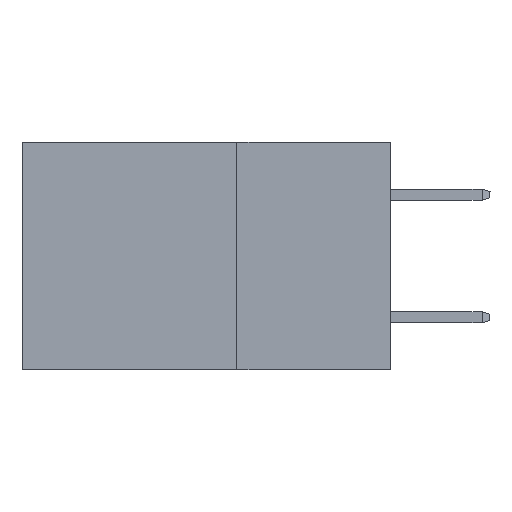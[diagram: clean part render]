
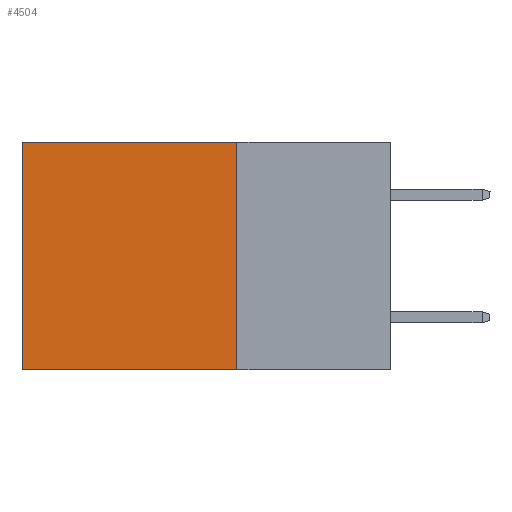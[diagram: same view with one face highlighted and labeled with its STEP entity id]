
A CAD part, left-side view. The second image highlights one B-rep face of the part: STEP entity #4504.
In plain terms, the highlighted planar face has unit normal (-1, 0, 0).
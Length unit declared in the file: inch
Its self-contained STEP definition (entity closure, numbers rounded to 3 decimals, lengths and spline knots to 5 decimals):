
#88 = VERTEX_POINT ( 'NONE', #887 ) ;
#652 = DIRECTION ( 'NONE',  ( 0., 1., 0. ) ) ;
#847 = LINE ( 'NONE', #7160, #8921 ) ;
#848 = VERTEX_POINT ( 'NONE', #3701 ) ;
#887 = CARTESIAN_POINT ( 'NONE',  ( 0.2875, 0.25, 0. ) ) ;
#898 = CARTESIAN_POINT ( 'NONE',  ( 0.2875, 0.25, -0.37 ) ) ;
#971 = ORIENTED_EDGE ( 'NONE', *, *, #4307, .T. ) ;
#2043 = EDGE_LOOP ( 'NONE', ( #971, #7208, #7688, #5482 ) ) ;
#2415 = CARTESIAN_POINT ( 'NONE',  ( 0.2875, 0.6, -0.37 ) ) ;
#2601 = LINE ( 'NONE', #8490, #6053 ) ;
#3211 = VECTOR ( 'NONE', #5764, 39.37008 ) ;
#3268 = DIRECTION ( 'NONE',  ( 0., 0., -1. ) ) ;
#3701 = CARTESIAN_POINT ( 'NONE',  ( 0.2875, 0.6, 0. ) ) ;
#4112 = VECTOR ( 'NONE', #3268, 39.37008 ) ;
#4233 = CARTESIAN_POINT ( 'NONE',  ( 0.2875, 0.25, 0. ) ) ;
#4261 = DIRECTION ( 'NONE',  ( 0., 0., -1. ) ) ;
#4307 = EDGE_CURVE ( 'NONE', #848, #8432, #2601, .T. ) ;
#4504 = ADVANCED_FACE ( 'NONE', ( #7251 ), #7919, .F. ) ;
#4534 = AXIS2_PLACEMENT_3D ( 'NONE', #9349, #6544, #4261 ) ;
#5391 = EDGE_CURVE ( 'NONE', #8497, #8432, #847, .T. ) ;
#5482 = ORIENTED_EDGE ( 'NONE', *, *, #9166, .T. ) ;
#5506 = LINE ( 'NONE', #6879, #4112 ) ;
#5708 = LINE ( 'NONE', #4233, #3211 ) ;
#5764 = DIRECTION ( 'NONE',  ( 0., 1., 0. ) ) ;
#6053 = VECTOR ( 'NONE', #9261, 39.37008 ) ;
#6544 = DIRECTION ( 'NONE',  ( 1., 0., 0. ) ) ;
#6879 = CARTESIAN_POINT ( 'NONE',  ( 0.2875, 0.25, 0. ) ) ;
#7160 = CARTESIAN_POINT ( 'NONE',  ( 0.2875, 0.25, -0.37 ) ) ;
#7208 = ORIENTED_EDGE ( 'NONE', *, *, #5391, .F. ) ;
#7251 = FACE_OUTER_BOUND ( 'NONE', #2043, .T. ) ;
#7688 = ORIENTED_EDGE ( 'NONE', *, *, #8614, .F. ) ;
#7919 = PLANE ( 'NONE',  #4534 ) ;
#8432 = VERTEX_POINT ( 'NONE', #2415 ) ;
#8490 = CARTESIAN_POINT ( 'NONE',  ( 0.2875, 0.6, 0. ) ) ;
#8497 = VERTEX_POINT ( 'NONE', #898 ) ;
#8614 = EDGE_CURVE ( 'NONE', #88, #8497, #5506, .T. ) ;
#8921 = VECTOR ( 'NONE', #652, 39.37008 ) ;
#9166 = EDGE_CURVE ( 'NONE', #88, #848, #5708, .T. ) ;
#9261 = DIRECTION ( 'NONE',  ( 0., 0., -1. ) ) ;
#9349 = CARTESIAN_POINT ( 'NONE',  ( 0.2875, 0.25, 0. ) ) ;
